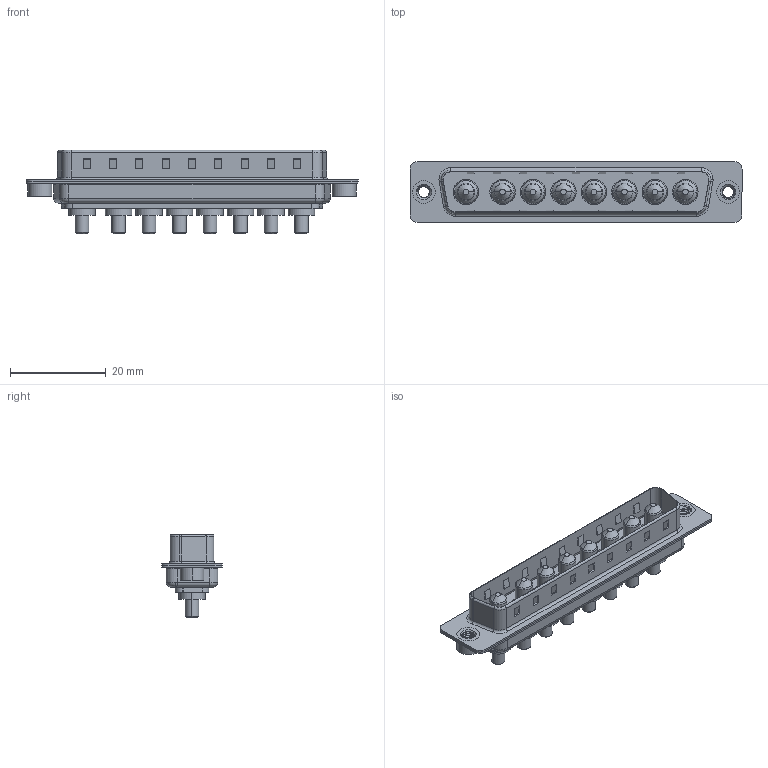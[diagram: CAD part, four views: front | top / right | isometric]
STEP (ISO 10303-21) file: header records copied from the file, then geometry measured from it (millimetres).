
FILE_DESCRIPTION (( 'STEP AP203' ), '1' );
FILE_NAME ('627-8W8-624-2NA.STEP', '2019-05-28T05:13:17', ( '' ), ( '' ), 'SwSTEP 2.0', 'SolidWorks 2016', '' );
FILE_SCHEMA (( 'CONFIG_CONTROL_DESIGN' ));
Length unit declared in the file: millimetre
Products named in the file (7): 627Combo Threaded Rivet_2; 627Combo Shell Rear_37 Contacts; 627Combo Threaded Rivet_A; 627Combo Shell Front_37 Contacts; 627Combo Housing_8W8; 627-8W8-624-2NA; Power Pin_20A S
Assembly tree (13 placements, depth 2):
  627-8W8-624-2NA
    627Combo Housing_8W8
    627Combo Shell Rear_37 Contacts
    627Combo Shell Front_37 Contacts
    627Combo Threaded Rivet_A
    Power Pin_20A S  x8
    627Combo Threaded Rivet_2
Bounding box: 69.3 x 12.6 x 17.4 mm (x, y, z)
Volume: 4330.9 mm3; surface area: 9229.6 mm2
Topology: 21 solids, 21 shells, 731 faces, 1734 edges, 1080 vertices
Faces by surface type: cylinder 294, plane 283, torus 66, cone 66, bspline 22
Entity records: 18735 total; most frequent: CARTESIAN_POINT 5886, DIRECTION 2555, ORIENTED_EDGE 2442, EDGE_CURVE 1221, AXIS2_PLACEMENT_3D 923, VERTEX_POINT 772, VECTOR 709, LINE 709
